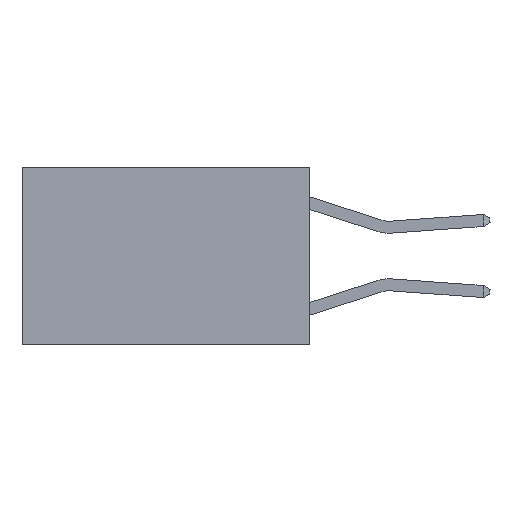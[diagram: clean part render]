
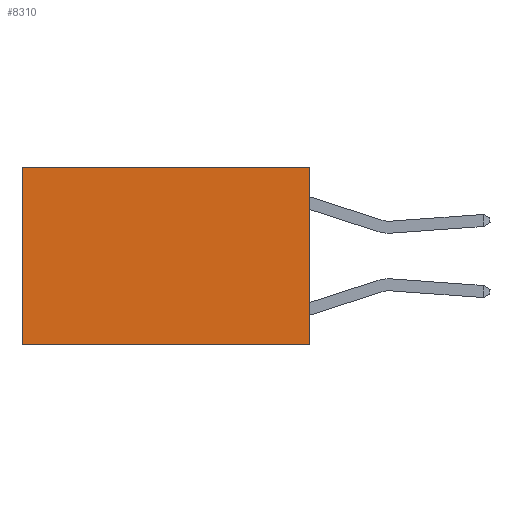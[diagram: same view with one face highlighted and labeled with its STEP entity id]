
A CAD part, left-side view. The second image highlights one B-rep face of the part: STEP entity #8310.
In plain terms, the highlighted planar face has unit normal (-1, 0, 0).
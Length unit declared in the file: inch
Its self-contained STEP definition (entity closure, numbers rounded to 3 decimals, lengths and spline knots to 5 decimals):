
#166 = CARTESIAN_POINT ( 'NONE',  ( 0.2625, 0., 0. ) ) ;
#851 = VERTEX_POINT ( 'NONE', #2051 ) ;
#908 = EDGE_CURVE ( 'NONE', #2604, #3882, #10105, .T. ) ;
#929 = DIRECTION ( 'NONE',  ( 0., 0., -1. ) ) ;
#1559 = VECTOR ( 'NONE', #7558, 39.37008 ) ;
#1647 = EDGE_CURVE ( 'NONE', #3882, #851, #9762, .T. ) ;
#1667 = DIRECTION ( 'NONE',  ( 1., 0., 0. ) ) ;
#2051 = CARTESIAN_POINT ( 'NONE',  ( 0.2625, 0.6, -0.37 ) ) ;
#2355 = CARTESIAN_POINT ( 'NONE',  ( 0.2625, 0.6, 0. ) ) ;
#2399 = ORIENTED_EDGE ( 'NONE', *, *, #1647, .T. ) ;
#2437 = CARTESIAN_POINT ( 'NONE',  ( 0.2625, 0., 0. ) ) ;
#2570 = VECTOR ( 'NONE', #929, 39.37008 ) ;
#2604 = VERTEX_POINT ( 'NONE', #2437 ) ;
#2704 = VERTEX_POINT ( 'NONE', #6850 ) ;
#2726 = CARTESIAN_POINT ( 'NONE',  ( 0.2625, 0.6, 0. ) ) ;
#2883 = ORIENTED_EDGE ( 'NONE', *, *, #8397, .F. ) ;
#3209 = CARTESIAN_POINT ( 'NONE',  ( 0.2625, 0., 0. ) ) ;
#3361 = AXIS2_PLACEMENT_3D ( 'NONE', #3209, #1667, #4735 ) ;
#3394 = LINE ( 'NONE', #166, #7427 ) ;
#3429 = ORIENTED_EDGE ( 'NONE', *, *, #908, .T. ) ;
#3578 = LINE ( 'NONE', #9825, #1559 ) ;
#3882 = VERTEX_POINT ( 'NONE', #2355 ) ;
#4702 = DIRECTION ( 'NONE',  ( 0., 1., 0. ) ) ;
#4735 = DIRECTION ( 'NONE',  ( 0., 0., -1. ) ) ;
#4851 = EDGE_CURVE ( 'NONE', #2604, #2704, #3394, .T. ) ;
#5492 = PLANE ( 'NONE',  #3361 ) ;
#6340 = CARTESIAN_POINT ( 'NONE',  ( 0.2625, 0., 0. ) ) ;
#6516 = VECTOR ( 'NONE', #4702, 39.37008 ) ;
#6850 = CARTESIAN_POINT ( 'NONE',  ( 0.2625, 0., -0.37 ) ) ;
#6902 = ORIENTED_EDGE ( 'NONE', *, *, #4851, .F. ) ;
#7427 = VECTOR ( 'NONE', #8651, 39.37008 ) ;
#7558 = DIRECTION ( 'NONE',  ( 0., 1., 0. ) ) ;
#7577 = EDGE_LOOP ( 'NONE', ( #2399, #2883, #6902, #3429 ) ) ;
#8310 = ADVANCED_FACE ( 'NONE', ( #8718 ), #5492, .F. ) ;
#8397 = EDGE_CURVE ( 'NONE', #2704, #851, #3578, .T. ) ;
#8651 = DIRECTION ( 'NONE',  ( 0., 0., -1. ) ) ;
#8718 = FACE_OUTER_BOUND ( 'NONE', #7577, .T. ) ;
#9762 = LINE ( 'NONE', #2726, #2570 ) ;
#9825 = CARTESIAN_POINT ( 'NONE',  ( 0.2625, 0., -0.37 ) ) ;
#10105 = LINE ( 'NONE', #6340, #6516 ) ;
